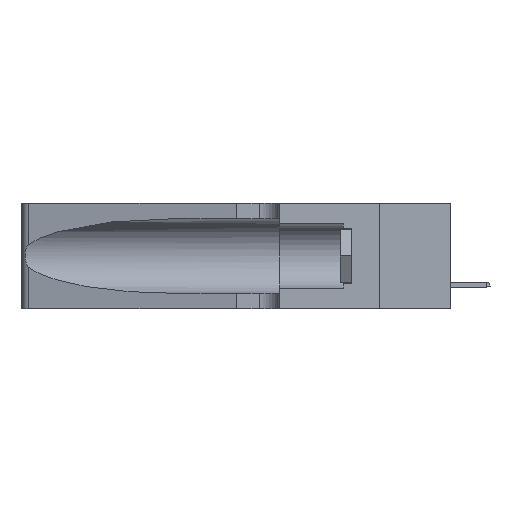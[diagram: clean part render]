
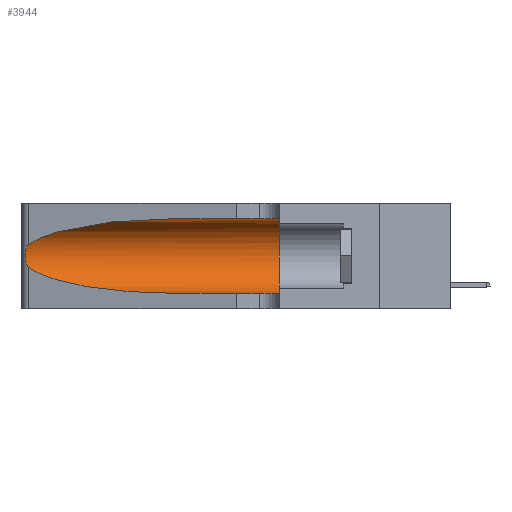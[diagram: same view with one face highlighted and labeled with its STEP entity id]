
A CAD part, left-side view. The second image highlights one B-rep face of the part: STEP entity #3944.
In plain terms, the highlighted cylindrical face has radius 3.308 mm (diameter 6.617 mm), a partial arc.
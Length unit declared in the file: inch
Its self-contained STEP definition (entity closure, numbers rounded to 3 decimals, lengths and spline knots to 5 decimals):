
#1298 = ORIENTED_EDGE ( 'NONE', *, *, #17328, .T. ) ;
#3073 = CARTESIAN_POINT ( 'NONE',  ( 0.25639, 1.23184, 0.21858 ) ) ;
#3342 = ORIENTED_EDGE ( 'NONE', *, *, #11594, .F. ) ;
#3790 = AXIS2_PLACEMENT_3D ( 'NONE', #28279, #31417, #4315 ) ;
#3944 = ADVANCED_FACE ( 'NONE', ( #34762 ), #5511, .F. ) ;
#4265 = VECTOR ( 'NONE', #28656, 39.37008 ) ;
#4315 = DIRECTION ( 'NONE',  ( 0., 0., 1. ) ) ;
#4442 = CARTESIAN_POINT ( 'NONE',  ( 0.2373, 1.15595, 0.08982 ) ) ;
#4781 = ORIENTED_EDGE ( 'NONE', *, *, #8461, .F. ) ;
#5199 = CARTESIAN_POINT ( 'NONE',  ( 0.1305, 0.35, 0.31525 ) ) ;
#5431 = VERTEX_POINT ( 'NONE', #23340 ) ;
#5511 = CYLINDRICAL_SURFACE ( 'NONE', #31732, 0.13025 ) ;
#5534 =( BOUNDED_CURVE ( )  B_SPLINE_CURVE ( 3, ( #22993, #29052, #26328, #20437 ),
 .UNSPECIFIED., .F., .T. ) 
 B_SPLINE_CURVE_WITH_KNOTS ( ( 4, 4 ),
 ( 1.5708, 2.84003 ),
 .UNSPECIFIED. ) 
 CURVE ( )  GEOMETRIC_REPRESENTATION_ITEM ( )  RATIONAL_B_SPLINE_CURVE ( ( 1., 0.87, 0.87, 1. ) ) 
 REPRESENTATION_ITEM ( '' )  );
#6106 = CARTESIAN_POINT ( 'NONE',  ( 0.1305, 1.61858, 0.05475 ) ) ;
#6481 = LINE ( 'NONE', #6106, #34943 ) ;
#8434 = DIRECTION ( 'NONE',  ( 0., 0., -1. ) ) ;
#8461 = EDGE_CURVE ( 'NONE', #10373, #16661, #11190, .T. ) ;
#8774 = CARTESIAN_POINT ( 'NONE',  ( 0.26075, 1.23896, 0.178 ) ) ;
#9082 = ORIENTED_EDGE ( 'NONE', *, *, #26770, .T. ) ;
#10150 = CARTESIAN_POINT ( 'NONE',  ( 0.1305, 0.72297, 0.05475 ) ) ;
#10373 = VERTEX_POINT ( 'NONE', #11942 ) ;
#10502 = CARTESIAN_POINT ( 'NONE',  ( 0.1305, 0.35, 0.05475 ) ) ;
#11190 = LINE ( 'NONE', #35135, #4265 ) ;
#11594 = EDGE_CURVE ( 'NONE', #16661, #21026, #37642, .T. ) ;
#11942 = CARTESIAN_POINT ( 'NONE',  ( 0.1305, 0.72297, 0.31525 ) ) ;
#12173 = B_SPLINE_CURVE_WITH_KNOTS ( 'NONE', 3,
 ( #33506, #35878, #3073, #21361, #15260, #23715, #35681, #8774, #33140, #24310, #33320, #32938, #18229, #30184 ),
 .UNSPECIFIED., .F., .F.,
 ( 4, 2, 2, 2, 2, 2, 4 ),
 ( 0., 0.00027, 0.00053, 0.00107, 0.0016, 0.00187, 0.00214 ),
 .UNSPECIFIED. ) ;
#12280 = ORIENTED_EDGE ( 'NONE', *, *, #14019, .T. ) ;
#14019 = EDGE_CURVE ( 'NONE', #33154, #17029, #12173, .T. ) ;
#14209 = CARTESIAN_POINT ( 'NONE',  ( 0.25487, 1.22718, 0.14631 ) ) ;
#15260 = CARTESIAN_POINT ( 'NONE',  ( 0.25854, 1.2359, 0.20912 ) ) ;
#15327 = DIRECTION ( 'NONE',  ( 0., -1., 0. ) ) ;
#16456 = CARTESIAN_POINT ( 'NONE',  ( 0.18966, 0.96281, 0.05475 ) ) ;
#16661 = VERTEX_POINT ( 'NONE', #5199 ) ;
#17029 = VERTEX_POINT ( 'NONE', #14209 ) ;
#17328 = EDGE_CURVE ( 'NONE', #10373, #33154, #5534, .T. ) ;
#18229 = CARTESIAN_POINT ( 'NONE',  ( 0.25555, 1.22993, 0.14849 ) ) ;
#18818 = EDGE_CURVE ( 'NONE', #5431, #21026, #6481, .T. ) ;
#20437 = CARTESIAN_POINT ( 'NONE',  ( 0.25487, 1.22718, 0.22369 ) ) ;
#20836 = EDGE_LOOP ( 'NONE', ( #1298, #12280, #9082, #34373, #3342, #4781 ) ) ;
#21026 = VERTEX_POINT ( 'NONE', #10502 ) ;
#21361 = CARTESIAN_POINT ( 'NONE',  ( 0.25787, 1.23484, 0.2124 ) ) ;
#22993 = CARTESIAN_POINT ( 'NONE',  ( 0.1305, 0.72297, 0.31525 ) ) ;
#23309 =( BOUNDED_CURVE ( )  B_SPLINE_CURVE ( 3, ( #34304, #4442, #16456, #10150 ),
 .UNSPECIFIED., .F., .T. ) 
 B_SPLINE_CURVE_WITH_KNOTS ( ( 4, 4 ),
 ( 3.44316, 4.71239 ),
 .UNSPECIFIED. ) 
 CURVE ( )  GEOMETRIC_REPRESENTATION_ITEM ( )  RATIONAL_B_SPLINE_CURVE ( ( 1., 0.87, 0.87, 1. ) ) 
 REPRESENTATION_ITEM ( '' )  );
#23340 = CARTESIAN_POINT ( 'NONE',  ( 0.1305, 0.72297, 0.05475 ) ) ;
#23573 = DIRECTION ( 'NONE',  ( 0., -1., 0. ) ) ;
#23715 = CARTESIAN_POINT ( 'NONE',  ( 0.26018, 1.23835, 0.19895 ) ) ;
#24310 = CARTESIAN_POINT ( 'NONE',  ( 0.25856, 1.23593, 0.16098 ) ) ;
#26328 = CARTESIAN_POINT ( 'NONE',  ( 0.2373, 1.15595, 0.28018 ) ) ;
#26770 = EDGE_CURVE ( 'NONE', #17029, #5431, #23309, .T. ) ;
#28279 = CARTESIAN_POINT ( 'NONE',  ( 0.1305, 0.35, 0.185 ) ) ;
#28656 = DIRECTION ( 'NONE',  ( 0., -1., 0. ) ) ;
#29052 = CARTESIAN_POINT ( 'NONE',  ( 0.18966, 0.96281, 0.31525 ) ) ;
#30184 = CARTESIAN_POINT ( 'NONE',  ( 0.25487, 1.22718, 0.14631 ) ) ;
#31417 = DIRECTION ( 'NONE',  ( 0., 1., 0. ) ) ;
#31732 = AXIS2_PLACEMENT_3D ( 'NONE', #35546, #23573, #8434 ) ;
#32938 = CARTESIAN_POINT ( 'NONE',  ( 0.25639, 1.23186, 0.15144 ) ) ;
#33140 = CARTESIAN_POINT ( 'NONE',  ( 0.26017, 1.23833, 0.17102 ) ) ;
#33154 = VERTEX_POINT ( 'NONE', #36001 ) ;
#33320 = CARTESIAN_POINT ( 'NONE',  ( 0.25789, 1.23486, 0.15765 ) ) ;
#33506 = CARTESIAN_POINT ( 'NONE',  ( 0.25487, 1.22718, 0.22369 ) ) ;
#34304 = CARTESIAN_POINT ( 'NONE',  ( 0.25487, 1.22718, 0.14631 ) ) ;
#34373 = ORIENTED_EDGE ( 'NONE', *, *, #18818, .T. ) ;
#34762 = FACE_OUTER_BOUND ( 'NONE', #20836, .T. ) ;
#34943 = VECTOR ( 'NONE', #15327, 39.37008 ) ;
#35135 = CARTESIAN_POINT ( 'NONE',  ( 0.1305, 1.61858, 0.31525 ) ) ;
#35546 = CARTESIAN_POINT ( 'NONE',  ( 0.1305, 1.61858, 0.185 ) ) ;
#35681 = CARTESIAN_POINT ( 'NONE',  ( 0.26075, 1.23896, 0.19203 ) ) ;
#35878 = CARTESIAN_POINT ( 'NONE',  ( 0.25555, 1.22994, 0.2215 ) ) ;
#36001 = CARTESIAN_POINT ( 'NONE',  ( 0.25487, 1.22718, 0.22369 ) ) ;
#37642 = CIRCLE ( 'NONE', #3790, 0.13025 ) ;
